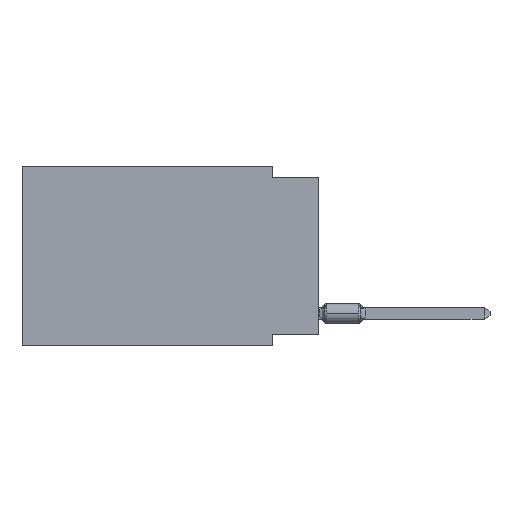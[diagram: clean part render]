
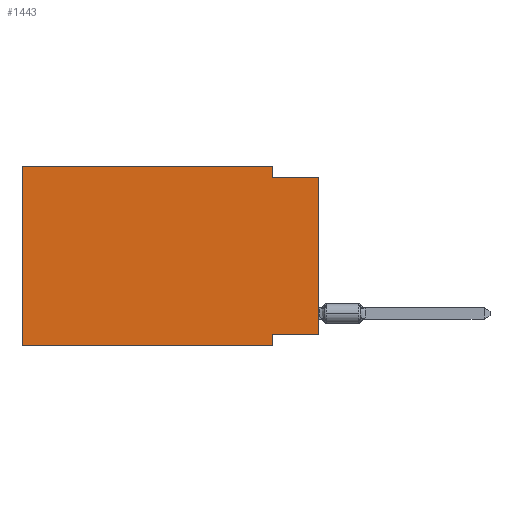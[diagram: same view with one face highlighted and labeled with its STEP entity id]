
A CAD part, left-side view. The second image highlights one B-rep face of the part: STEP entity #1443.
In plain terms, the highlighted planar face has unit normal (-1, 0, 0).
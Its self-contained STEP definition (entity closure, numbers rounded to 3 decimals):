
#189 = VERTEX_POINT ( 'NONE', #7206 ) ;
#226 = LINE ( 'NONE', #4653, #10872 ) ;
#472 = EDGE_CURVE ( 'NONE', #5124, #7341, #226, .T. ) ;
#615 = EDGE_LOOP ( 'NONE', ( #24045, #7059, #18509, #7907, #23285, #12101, #24783, #23594 ) ) ;
#880 = LINE ( 'NONE', #13059, #5126 ) ;
#1051 = CARTESIAN_POINT ( 'NONE',  ( 0., 16.383, 0. ) ) ;
#1443 = ADVANCED_FACE ( 'NONE', ( #24285 ), #8787, .F. ) ;
#2938 = DIRECTION ( 'NONE',  ( 0., 0., -1. ) ) ;
#4210 = VECTOR ( 'NONE', #23866, 1000. ) ;
#4381 = CARTESIAN_POINT ( 'NONE',  ( 0., 2.54, -9.906 ) ) ;
#4653 = CARTESIAN_POINT ( 'NONE',  ( 0., 16.383, -9.906 ) ) ;
#4679 = CARTESIAN_POINT ( 'NONE',  ( 0., 16.383, 0. ) ) ;
#5124 = VERTEX_POINT ( 'NONE', #17288 ) ;
#5126 = VECTOR ( 'NONE', #8630, 1000. ) ;
#5469 = VECTOR ( 'NONE', #8063, 1000. ) ;
#5908 = LINE ( 'NONE', #4381, #5469 ) ;
#6749 = LINE ( 'NONE', #16654, #16717 ) ;
#7032 = VECTOR ( 'NONE', #13469, 1000. ) ;
#7059 = ORIENTED_EDGE ( 'NONE', *, *, #24491, .F. ) ;
#7206 = CARTESIAN_POINT ( 'NONE',  ( 0., 2.54, 0. ) ) ;
#7341 = VERTEX_POINT ( 'NONE', #21310 ) ;
#7907 = ORIENTED_EDGE ( 'NONE', *, *, #22221, .F. ) ;
#8063 = DIRECTION ( 'NONE',  ( 0., 0., -1. ) ) ;
#8472 = AXIS2_PLACEMENT_3D ( 'NONE', #1051, #22368, #2938 ) ;
#8630 = DIRECTION ( 'NONE',  ( 0., 0., -1. ) ) ;
#8787 = PLANE ( 'NONE',  #8472 ) ;
#8896 = CARTESIAN_POINT ( 'NONE',  ( 0., 16.383, 0. ) ) ;
#9241 = EDGE_CURVE ( 'NONE', #21016, #10613, #23304, .T. ) ;
#9583 = CARTESIAN_POINT ( 'NONE',  ( 0., 0., -9.271 ) ) ;
#10613 = VERTEX_POINT ( 'NONE', #24869 ) ;
#10872 = VECTOR ( 'NONE', #16207, 1000. ) ;
#11237 = EDGE_CURVE ( 'NONE', #21016, #12028, #17132, .T. ) ;
#12028 = VERTEX_POINT ( 'NONE', #20767 ) ;
#12101 = ORIENTED_EDGE ( 'NONE', *, *, #472, .T. ) ;
#13059 = CARTESIAN_POINT ( 'NONE',  ( 0., 2.54, 0. ) ) ;
#13469 = DIRECTION ( 'NONE',  ( 0., 0., 1. ) ) ;
#13692 = CARTESIAN_POINT ( 'NONE',  ( 0., 0., -9.271 ) ) ;
#14320 = LINE ( 'NONE', #4679, #4210 ) ;
#15039 = EDGE_CURVE ( 'NONE', #189, #21163, #880, .T. ) ;
#15171 = DIRECTION ( 'NONE',  ( 0., 1., 0. ) ) ;
#16207 = DIRECTION ( 'NONE',  ( 0., -1., 0. ) ) ;
#16435 = EDGE_CURVE ( 'NONE', #5124, #21922, #19920, .T. ) ;
#16654 = CARTESIAN_POINT ( 'NONE',  ( 0., 0., -0.635 ) ) ;
#16717 = VECTOR ( 'NONE', #24406, 1000. ) ;
#16896 = DIRECTION ( 'NONE',  ( 0., 0., 1. ) ) ;
#17132 = LINE ( 'NONE', #17388, #22903 ) ;
#17288 = CARTESIAN_POINT ( 'NONE',  ( 0., 16.383, -9.906 ) ) ;
#17374 = EDGE_CURVE ( 'NONE', #10613, #7341, #5908, .T. ) ;
#17388 = CARTESIAN_POINT ( 'NONE',  ( 0., 0., 0. ) ) ;
#18509 = ORIENTED_EDGE ( 'NONE', *, *, #15039, .F. ) ;
#19920 = LINE ( 'NONE', #21933, #7032 ) ;
#20767 = CARTESIAN_POINT ( 'NONE',  ( 0., 0., -0.635 ) ) ;
#21016 = VERTEX_POINT ( 'NONE', #13692 ) ;
#21163 = VERTEX_POINT ( 'NONE', #24713 ) ;
#21310 = CARTESIAN_POINT ( 'NONE',  ( 0., 2.54, -9.906 ) ) ;
#21922 = VERTEX_POINT ( 'NONE', #8896 ) ;
#21933 = CARTESIAN_POINT ( 'NONE',  ( 0., 16.383, 0. ) ) ;
#22221 = EDGE_CURVE ( 'NONE', #21922, #189, #14320, .T. ) ;
#22368 = DIRECTION ( 'NONE',  ( 1., 0., 0. ) ) ;
#22903 = VECTOR ( 'NONE', #16896, 1000. ) ;
#23192 = VECTOR ( 'NONE', #15171, 1000. ) ;
#23285 = ORIENTED_EDGE ( 'NONE', *, *, #16435, .F. ) ;
#23304 = LINE ( 'NONE', #9583, #23192 ) ;
#23594 = ORIENTED_EDGE ( 'NONE', *, *, #9241, .F. ) ;
#23866 = DIRECTION ( 'NONE',  ( 0., -1., 0. ) ) ;
#24045 = ORIENTED_EDGE ( 'NONE', *, *, #11237, .T. ) ;
#24285 = FACE_OUTER_BOUND ( 'NONE', #615, .T. ) ;
#24406 = DIRECTION ( 'NONE',  ( 0., -1., 0. ) ) ;
#24491 = EDGE_CURVE ( 'NONE', #21163, #12028, #6749, .T. ) ;
#24713 = CARTESIAN_POINT ( 'NONE',  ( 0., 2.54, -0.635 ) ) ;
#24783 = ORIENTED_EDGE ( 'NONE', *, *, #17374, .F. ) ;
#24869 = CARTESIAN_POINT ( 'NONE',  ( 0., 2.54, -9.271 ) ) ;
